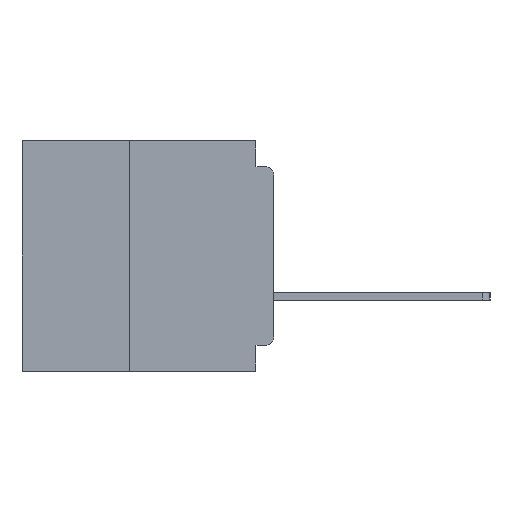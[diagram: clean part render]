
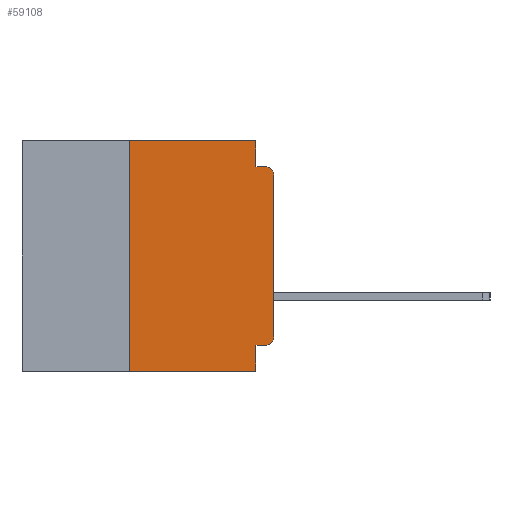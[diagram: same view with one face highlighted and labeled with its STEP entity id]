
A CAD part, left-side view. The second image highlights one B-rep face of the part: STEP entity #59108.
In plain terms, the highlighted planar face has unit normal (-1, 0, 0).
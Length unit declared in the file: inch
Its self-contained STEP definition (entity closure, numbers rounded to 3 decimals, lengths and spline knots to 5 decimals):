
#108 = LINE ( 'NONE', #41501, #11586 ) ;
#1411 = CARTESIAN_POINT ( 'NONE',  ( 0., 0.25, 0. ) ) ;
#2064 = DIRECTION ( 'NONE',  ( 0., -1., 0. ) ) ;
#2070 = LINE ( 'NONE', #59223, #36436 ) ;
#2335 = VECTOR ( 'NONE', #50299, 39.37008 ) ;
#3586 = AXIS2_PLACEMENT_3D ( 'NONE', #55741, #26714, #60613 ) ;
#5001 = CARTESIAN_POINT ( 'NONE',  ( 0., 0.437, 0. ) ) ;
#6838 = DIRECTION ( 'NONE',  ( -1., 0., 0. ) ) ;
#6857 = VERTEX_POINT ( 'NONE', #38625 ) ;
#8093 = VERTEX_POINT ( 'NONE', #18862 ) ;
#8414 = DIRECTION ( 'NONE',  ( 0., 0., 1. ) ) ;
#8480 = DIRECTION ( 'NONE',  ( 0., 0., -1. ) ) ;
#9097 = ORIENTED_EDGE ( 'NONE', *, *, #62049, .F. ) ;
#10451 = VERTEX_POINT ( 'NONE', #52544 ) ;
#11586 = VECTOR ( 'NONE', #12300, 39.37008 ) ;
#12192 = ORIENTED_EDGE ( 'NONE', *, *, #44780, .T. ) ;
#12300 = DIRECTION ( 'NONE',  ( 0., 1., 0. ) ) ;
#12726 = FACE_OUTER_BOUND ( 'NONE', #58771, .T. ) ;
#13176 = CARTESIAN_POINT ( 'NONE',  ( 0., 0.031, 0. ) ) ;
#13498 = DIRECTION ( 'NONE',  ( 0., 0., -1. ) ) ;
#13577 = EDGE_CURVE ( 'NONE', #10451, #39451, #2070, .T. ) ;
#13780 = LINE ( 'NONE', #16292, #2335 ) ;
#13789 = EDGE_CURVE ( 'NONE', #43566, #20947, #61363, .T. ) ;
#14196 = CIRCLE ( 'NONE', #30002, 0.015 ) ;
#14233 = EDGE_CURVE ( 'NONE', #62629, #55728, #14196, .T. ) ;
#14245 = VECTOR ( 'NONE', #13498, 39.37008 ) ;
#14917 = CARTESIAN_POINT ( 'NONE',  ( 0., 0.25, -0.4 ) ) ;
#15032 = DIRECTION ( 'NONE',  ( 1., 0., 0. ) ) ;
#15409 = AXIS2_PLACEMENT_3D ( 'NONE', #5001, #15032, #49035 ) ;
#16292 = CARTESIAN_POINT ( 'NONE',  ( 0., 0.437, 0. ) ) ;
#17854 = VECTOR ( 'NONE', #2064, 39.37008 ) ;
#18238 = CARTESIAN_POINT ( 'NONE',  ( 0., 0., 0. ) ) ;
#18862 = CARTESIAN_POINT ( 'NONE',  ( 0., 0., -0.06 ) ) ;
#18939 = CARTESIAN_POINT ( 'NONE',  ( 0., 0., -0.34 ) ) ;
#19169 = EDGE_CURVE ( 'NONE', #48787, #51444, #35373, .T. ) ;
#19376 = LINE ( 'NONE', #26441, #17854 ) ;
#20353 = DIRECTION ( 'NONE',  ( 0., -1., 0. ) ) ;
#20947 = VERTEX_POINT ( 'NONE', #26903 ) ;
#22404 = VECTOR ( 'NONE', #58680, 39.37008 ) ;
#23952 = ORIENTED_EDGE ( 'NONE', *, *, #41050, .T. ) ;
#26441 = CARTESIAN_POINT ( 'NONE',  ( 0., 0.437, -0.4 ) ) ;
#26714 = DIRECTION ( 'NONE',  ( -1., 0., 0. ) ) ;
#26903 = CARTESIAN_POINT ( 'NONE',  ( 0., 0.031, -0.4 ) ) ;
#28456 = CARTESIAN_POINT ( 'NONE',  ( 0., 0.031, -0.355 ) ) ;
#30002 = AXIS2_PLACEMENT_3D ( 'NONE', #36099, #6838, #40966 ) ;
#31098 = EDGE_CURVE ( 'NONE', #8093, #39451, #34941, .T. ) ;
#31696 = ORIENTED_EDGE ( 'NONE', *, *, #37989, .F. ) ;
#34473 = PLANE ( 'NONE',  #15409 ) ;
#34911 = VECTOR ( 'NONE', #8414, 39.37008 ) ;
#34941 = CIRCLE ( 'NONE', #3586, 0.015 ) ;
#35373 = LINE ( 'NONE', #14917, #22404 ) ;
#36099 = CARTESIAN_POINT ( 'NONE',  ( 0., 0.015, -0.34 ) ) ;
#36436 = VECTOR ( 'NONE', #20353, 39.37008 ) ;
#36442 = LINE ( 'NONE', #18238, #34911 ) ;
#37989 = EDGE_CURVE ( 'NONE', #62629, #43566, #108, .T. ) ;
#38625 = CARTESIAN_POINT ( 'NONE',  ( 0., 0.031, 0. ) ) ;
#39451 = VERTEX_POINT ( 'NONE', #47830 ) ;
#39567 = ORIENTED_EDGE ( 'NONE', *, *, #31098, .T. ) ;
#40966 = DIRECTION ( 'NONE',  ( 0., 0., -1. ) ) ;
#41050 = EDGE_CURVE ( 'NONE', #48787, #20947, #19376, .T. ) ;
#41501 = CARTESIAN_POINT ( 'NONE',  ( 0., 0., -0.355 ) ) ;
#42669 = CARTESIAN_POINT ( 'NONE',  ( 0., 0.031, -0.4 ) ) ;
#43566 = VERTEX_POINT ( 'NONE', #28456 ) ;
#43800 = ORIENTED_EDGE ( 'NONE', *, *, #14233, .T. ) ;
#43897 = CARTESIAN_POINT ( 'NONE',  ( 0., 0.25, -0.4 ) ) ;
#44780 = EDGE_CURVE ( 'NONE', #55728, #8093, #36442, .T. ) ;
#45315 = CARTESIAN_POINT ( 'NONE',  ( 0., 0.015, -0.355 ) ) ;
#47830 = CARTESIAN_POINT ( 'NONE',  ( 0., 0.015, -0.045 ) ) ;
#48787 = VERTEX_POINT ( 'NONE', #43897 ) ;
#49035 = DIRECTION ( 'NONE',  ( 0., 0., -1. ) ) ;
#50213 = EDGE_CURVE ( 'NONE', #51444, #6857, #13780, .T. ) ;
#50299 = DIRECTION ( 'NONE',  ( 0., -1., 0. ) ) ;
#50462 = LINE ( 'NONE', #13176, #61807 ) ;
#51444 = VERTEX_POINT ( 'NONE', #1411 ) ;
#52544 = CARTESIAN_POINT ( 'NONE',  ( 0., 0.031, -0.045 ) ) ;
#54518 = ORIENTED_EDGE ( 'NONE', *, *, #13789, .F. ) ;
#55728 = VERTEX_POINT ( 'NONE', #18939 ) ;
#55741 = CARTESIAN_POINT ( 'NONE',  ( 0., 0.015, -0.06 ) ) ;
#58415 = ORIENTED_EDGE ( 'NONE', *, *, #13577, .F. ) ;
#58680 = DIRECTION ( 'NONE',  ( 0., 0., 1. ) ) ;
#58690 = ORIENTED_EDGE ( 'NONE', *, *, #50213, .F. ) ;
#58771 = EDGE_LOOP ( 'NONE', ( #12192, #39567, #58415, #9097, #58690, #60432, #23952, #54518, #31696, #43800 ) ) ;
#59108 = ADVANCED_FACE ( 'NONE', ( #12726 ), #34473, .F. ) ;
#59223 = CARTESIAN_POINT ( 'NONE',  ( 0., 0., -0.045 ) ) ;
#60432 = ORIENTED_EDGE ( 'NONE', *, *, #19169, .F. ) ;
#60613 = DIRECTION ( 'NONE',  ( 0., 0., -1. ) ) ;
#61363 = LINE ( 'NONE', #42669, #14245 ) ;
#61807 = VECTOR ( 'NONE', #8480, 39.37008 ) ;
#62049 = EDGE_CURVE ( 'NONE', #6857, #10451, #50462, .T. ) ;
#62629 = VERTEX_POINT ( 'NONE', #45315 ) ;
